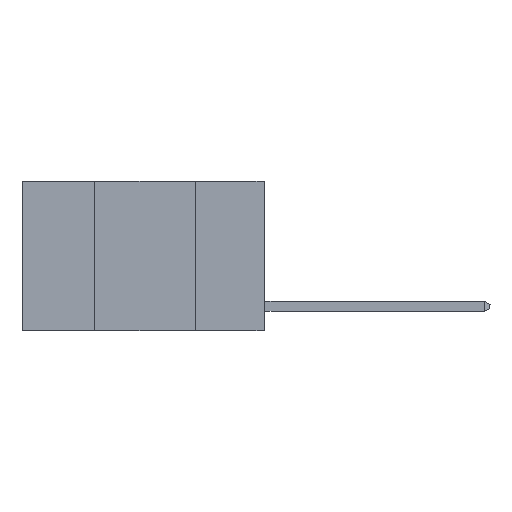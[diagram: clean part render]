
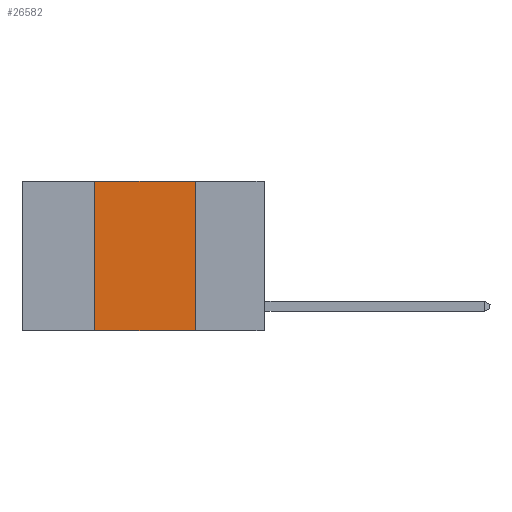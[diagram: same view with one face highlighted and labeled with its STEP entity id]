
A CAD part, left-side view. The second image highlights one B-rep face of the part: STEP entity #26582.
In plain terms, the highlighted planar face has unit normal (-1, 0, 0).
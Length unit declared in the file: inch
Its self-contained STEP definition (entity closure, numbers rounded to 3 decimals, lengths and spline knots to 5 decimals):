
#733 = VERTEX_POINT ( 'NONE', #19951 ) ;
#1006 = DIRECTION ( 'NONE',  ( 0., 0., -1. ) ) ;
#1169 = DIRECTION ( 'NONE',  ( 0., -1., 0. ) ) ;
#1574 = DIRECTION ( 'NONE',  ( 0., -1., 0. ) ) ;
#2374 = VERTEX_POINT ( 'NONE', #4232 ) ;
#3999 = CARTESIAN_POINT ( 'NONE',  ( 0., 0.17, -0.37 ) ) ;
#4232 = CARTESIAN_POINT ( 'NONE',  ( 0., 0.42, -0.37 ) ) ;
#4885 = VERTEX_POINT ( 'NONE', #3999 ) ;
#5050 = VERTEX_POINT ( 'NONE', #5144 ) ;
#5144 = CARTESIAN_POINT ( 'NONE',  ( 0., 0.17, 0. ) ) ;
#7775 = ORIENTED_EDGE ( 'NONE', *, *, #13533, .F. ) ;
#8230 = LINE ( 'NONE', #16913, #25349 ) ;
#8321 = EDGE_CURVE ( 'NONE', #2374, #4885, #8230, .T. ) ;
#9439 = FACE_OUTER_BOUND ( 'NONE', #12483, .T. ) ;
#10560 = VECTOR ( 'NONE', #1169, 39.37008 ) ;
#11219 = LINE ( 'NONE', #20056, #20577 ) ;
#11915 = LINE ( 'NONE', #27389, #21832 ) ;
#12483 = EDGE_LOOP ( 'NONE', ( #14982, #7775, #24838, #16861 ) ) ;
#12658 = CARTESIAN_POINT ( 'NONE',  ( 0., 0.6, 0. ) ) ;
#13512 = DIRECTION ( 'NONE',  ( 0., 0., -1. ) ) ;
#13533 = EDGE_CURVE ( 'NONE', #733, #5050, #14207, .T. ) ;
#14207 = LINE ( 'NONE', #12658, #10560 ) ;
#14318 = DIRECTION ( 'NONE',  ( 1., 0., 0. ) ) ;
#14982 = ORIENTED_EDGE ( 'NONE', *, *, #22476, .F. ) ;
#16355 = CARTESIAN_POINT ( 'NONE',  ( 0., 0.6, 0. ) ) ;
#16861 = ORIENTED_EDGE ( 'NONE', *, *, #8321, .T. ) ;
#16913 = CARTESIAN_POINT ( 'NONE',  ( 0., 0.6, -0.37 ) ) ;
#18415 = PLANE ( 'NONE',  #18843 ) ;
#18843 = AXIS2_PLACEMENT_3D ( 'NONE', #16355, #14318, #1006 ) ;
#19951 = CARTESIAN_POINT ( 'NONE',  ( 0., 0.42, 0. ) ) ;
#20056 = CARTESIAN_POINT ( 'NONE',  ( 0., 0.17, 0. ) ) ;
#20577 = VECTOR ( 'NONE', #13512, 39.37008 ) ;
#20722 = EDGE_CURVE ( 'NONE', #2374, #733, #11915, .T. ) ;
#21832 = VECTOR ( 'NONE', #24804, 39.37008 ) ;
#22476 = EDGE_CURVE ( 'NONE', #5050, #4885, #11219, .T. ) ;
#24804 = DIRECTION ( 'NONE',  ( 0., 0., 1. ) ) ;
#24838 = ORIENTED_EDGE ( 'NONE', *, *, #20722, .F. ) ;
#25349 = VECTOR ( 'NONE', #1574, 39.37008 ) ;
#26582 = ADVANCED_FACE ( 'NONE', ( #9439 ), #18415, .F. ) ;
#27389 = CARTESIAN_POINT ( 'NONE',  ( 0., 0.42, 0. ) ) ;
